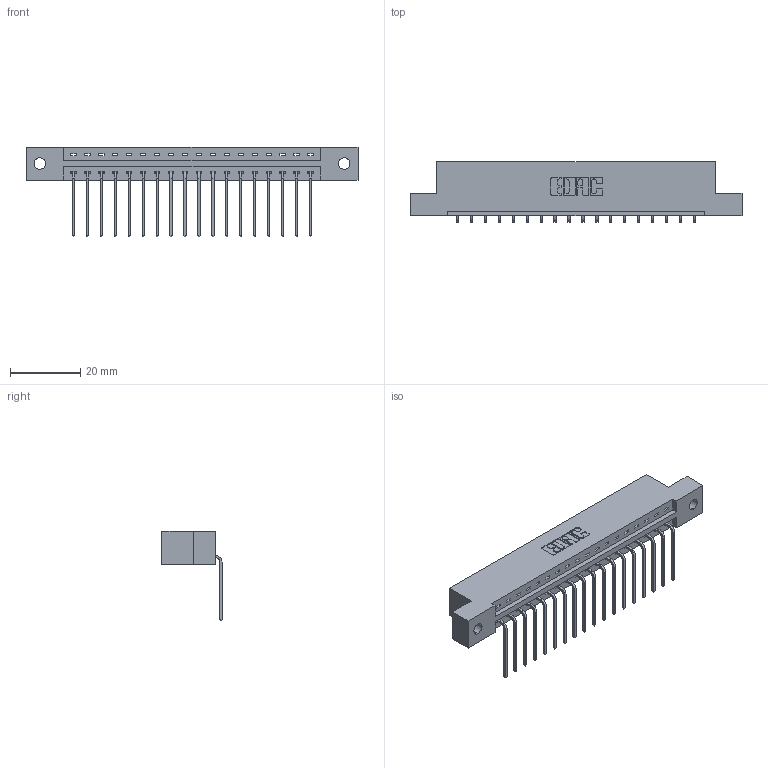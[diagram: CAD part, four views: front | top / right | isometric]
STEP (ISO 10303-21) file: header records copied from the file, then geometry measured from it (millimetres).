
FILE_DESCRIPTION (( 'STEP AP203' ), '1' );
FILE_NAME ('337-018-559-102.STEP', '2019-09-28T20:37:42', ( '' ), ( '' ), 'SwSTEP 2.0', 'SolidWorks 2016', '' );
FILE_SCHEMA (( 'CONFIG_CONTROL_DESIGN' ));
Length unit declared in the file: inch
Products named in the file (3): 337 Part_Flush Mounting Lugs - 0.128 Dia; 345-292-001_558 559 Tail - 1; 337-018-559-102
Assembly tree (19 placements, depth 2):
  337-018-559-102
    337 Part_Flush Mounting Lugs - 0.128 Dia
    345-292-001_558 559 Tail - 1  x18
Bounding box: 94.34 x 17.09 x 25.53 mm (x, y, z)
Volume: 9527.6 mm3; surface area: 9810.7 mm2
Topology: 19 solids, 19 shells, 1266 faces, 3803 edges, 2510 vertices
Faces by surface type: plane 934, cylinder 332
Entity records: 16571 total; most frequent: CARTESIAN_POINT 2892, ORIENTED_EDGE 2846, DIRECTION 2483, EDGE_CURVE 1423, VECTOR 1295, LINE 1295, VERTEX_POINT 946, AXIS2_PLACEMENT_3D 594
